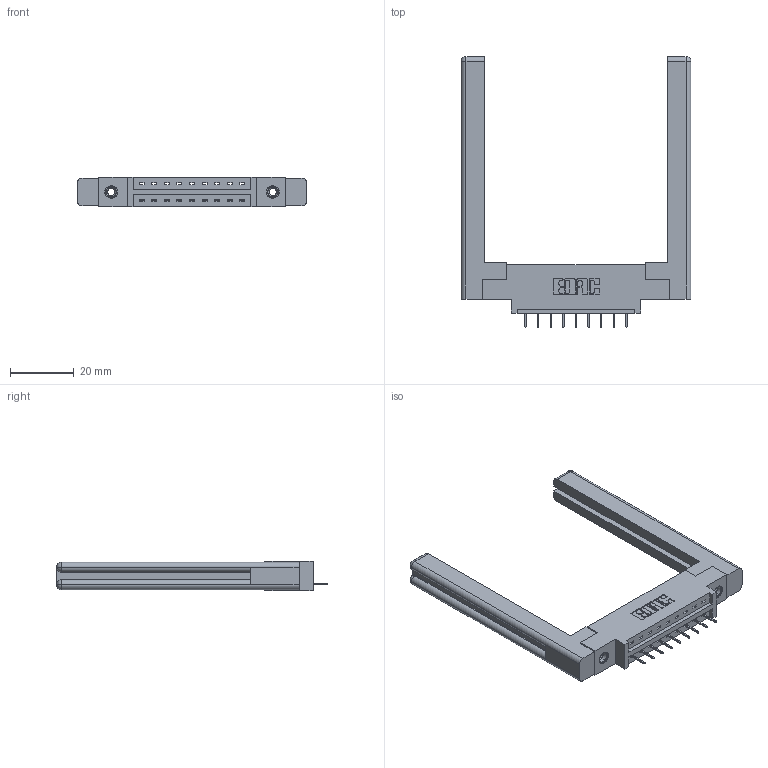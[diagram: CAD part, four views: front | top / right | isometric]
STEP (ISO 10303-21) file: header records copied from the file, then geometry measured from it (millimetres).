
FILE_DESCRIPTION (( 'STEP AP203' ), '1' );
FILE_NAME ('337-009-524-658.STEP', '2019-09-27T20:08:27', ( '' ), ( '' ), 'SwSTEP 2.0', 'SolidWorks 2016', '' );
FILE_SCHEMA (( 'CONFIG_CONTROL_DESIGN' ));
Length unit declared in the file: inch
Products named in the file (5): 337-009-524-658; 307-220-058; 345-250-001_345-250-001-102; 337 Part_0.170 Offset - 0.156 Dia-TI; 345-292-001_345-293-124
Assembly tree (14 placements, depth 2):
  337-009-524-658
    337 Part_0.170 Offset - 0.156 Dia-TI
    345-292-001_345-293-124  x9
    345-250-001_345-250-001-102  x2
    307-220-058  x2
Bounding box: 72.29 x 85.1 x 9.4 mm (x, y, z)
Volume: 14109.3 mm3; surface area: 12180.1 mm2
Topology: 14 solids, 14 shells, 854 faces, 2405 edges, 1554 vertices
Faces by surface type: plane 626, cylinder 204, cone 12, torus 12
Entity records: 13798 total; most frequent: CARTESIAN_POINT 2400, ORIENTED_EDGE 2284, DIRECTION 2108, EDGE_CURVE 1142, VECTOR 970, LINE 970, VERTEX_POINT 750, AXIS2_PLACEMENT_3D 569
